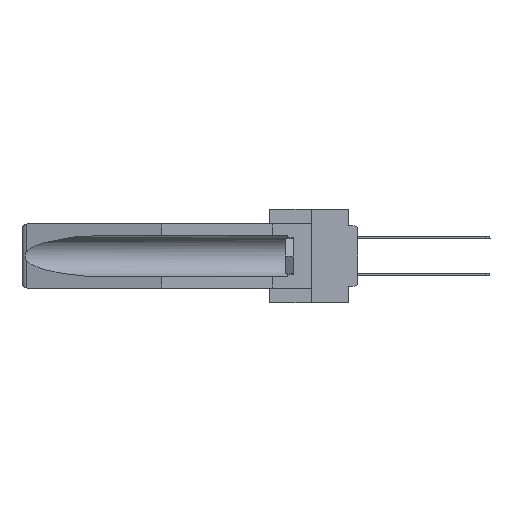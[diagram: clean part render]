
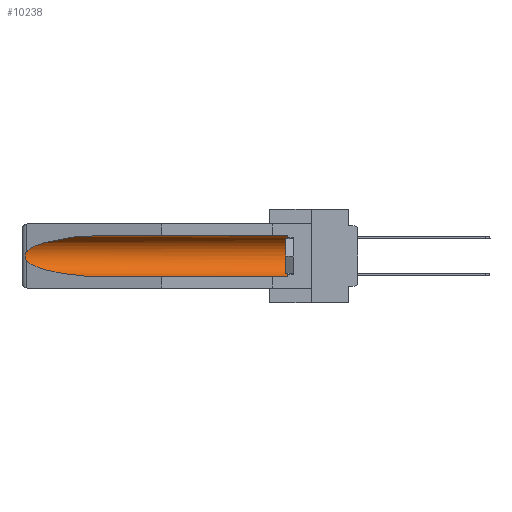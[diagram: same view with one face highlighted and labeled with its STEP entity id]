
A CAD part, left-side view. The second image highlights one B-rep face of the part: STEP entity #10238.
In plain terms, the highlighted cylindrical face has radius 2.857 mm (diameter 5.715 mm), a partial arc.
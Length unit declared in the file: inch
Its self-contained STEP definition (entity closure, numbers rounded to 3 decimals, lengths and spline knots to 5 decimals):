
#46 = EDGE_LOOP ( 'NONE', ( #25055, #23466, #17663, #6722, #11705, #9117 ) ) ;
#323 = AXIS2_PLACEMENT_3D ( 'NONE', #9166, #14554, #29353 ) ;
#663 = VECTOR ( 'NONE', #30171, 39.37008 ) ;
#1016 = CARTESIAN_POINT ( 'NONE',  ( 0.26537, 1.52718, -0.19328 ) ) ;
#2101 = DIRECTION ( 'NONE',  ( 0., 1., 0. ) ) ;
#3314 = CARTESIAN_POINT ( 'NONE',  ( 0.155, -0.30754, -0.284 ) ) ;
#3379 = VECTOR ( 'NONE', #2101, 39.37008 ) ;
#4280 =( BOUNDED_CURVE ( )  B_SPLINE_CURVE ( 3, ( #18358, #13815, #28750, #16086 ),
 .UNSPECIFIED., .F., .T. ) 
 B_SPLINE_CURVE_WITH_KNOTS ( ( 4, 4 ),
 ( 4.71239, 6.08839 ),
 .UNSPECIFIED. ) 
 CURVE ( )  GEOMETRIC_REPRESENTATION_ITEM ( )  RATIONAL_B_SPLINE_CURVE ( ( 1., 0.848, 0.848, 1. ) ) 
 REPRESENTATION_ITEM ( '' )  );
#4795 = CARTESIAN_POINT ( 'NONE',  ( 0.2675, 1.53308, -0.17534 ) ) ;
#5917 = EDGE_CURVE ( 'NONE', #19078, #24408, #18412, .T. ) ;
#6722 = ORIENTED_EDGE ( 'NONE', *, *, #12172, .F. ) ;
#9117 = ORIENTED_EDGE ( 'NONE', *, *, #14788, .T. ) ;
#9166 = CARTESIAN_POINT ( 'NONE',  ( 0.155, 0.126, -0.1715 ) ) ;
#10238 = ADVANCED_FACE ( 'NONE', ( #21677 ), #19865, .F. ) ;
#11245 = CARTESIAN_POINT ( 'NONE',  ( 0.21114, 1.30732, -0.284 ) ) ;
#11557 = CARTESIAN_POINT ( 'NONE',  ( 0.26537, 1.52718, -0.19328 ) ) ;
#11705 = ORIENTED_EDGE ( 'NONE', *, *, #15623, .T. ) ;
#12172 = EDGE_CURVE ( 'NONE', #29720, #23252, #22538, .T. ) ;
#13815 = CARTESIAN_POINT ( 'NONE',  ( 0.21114, 1.30732, -0.059 ) ) ;
#14375 = CIRCLE ( 'NONE', #323, 0.1125 ) ;
#14478 = LINE ( 'NONE', #14799, #3379 ) ;
#14554 = DIRECTION ( 'NONE',  ( 0., -1., 0. ) ) ;
#14788 = EDGE_CURVE ( 'NONE', #26849, #15546, #14478, .T. ) ;
#14799 = CARTESIAN_POINT ( 'NONE',  ( 0.155, -0.30754, -0.059 ) ) ;
#15546 = VERTEX_POINT ( 'NONE', #28231 ) ;
#15623 = EDGE_CURVE ( 'NONE', #29720, #26849, #14375, .T. ) ;
#16086 = CARTESIAN_POINT ( 'NONE',  ( 0.26537, 1.52718, -0.14972 ) ) ;
#16120 = CARTESIAN_POINT ( 'NONE',  ( 0.155, 1.07973, -0.284 ) ) ;
#16335 = EDGE_CURVE ( 'NONE', #15546, #19078, #4280, .T. ) ;
#17203 = CARTESIAN_POINT ( 'NONE',  ( 0.26654, 1.53092, -0.15636 ) ) ;
#17396 = CARTESIAN_POINT ( 'NONE',  ( 0.155, 1.07973, -0.284 ) ) ;
#17663 = ORIENTED_EDGE ( 'NONE', *, *, #23042, .T. ) ;
#17802 =( BOUNDED_CURVE ( )  B_SPLINE_CURVE ( 3, ( #11557, #26660, #11245, #16120 ),
 .UNSPECIFIED., .F., .T. ) 
 B_SPLINE_CURVE_WITH_KNOTS ( ( 4, 4 ),
 ( 0.1948, 1.5708 ),
 .UNSPECIFIED. ) 
 CURVE ( )  GEOMETRIC_REPRESENTATION_ITEM ( )  RATIONAL_B_SPLINE_CURVE ( ( 1., 0.848, 0.848, 1. ) ) 
 REPRESENTATION_ITEM ( '' )  );
#18046 = CARTESIAN_POINT ( 'NONE',  ( 0.155, 0.126, -0.059 ) ) ;
#18358 = CARTESIAN_POINT ( 'NONE',  ( 0.155, 1.07973, -0.059 ) ) ;
#18412 = B_SPLINE_CURVE_WITH_KNOTS ( 'NONE', 3,
 ( #20285, #22400, #17203, #27116, #19973, #4795, #25145, #22559, #27756, #22239 ),
 .UNSPECIFIED., .F., .F.,
 ( 4, 2, 2, 2, 4 ),
 ( 0., 0.00029, 0.00058, 0.00087, 0.00117 ),
 .UNSPECIFIED. ) ;
#19078 = VERTEX_POINT ( 'NONE', #19214 ) ;
#19214 = CARTESIAN_POINT ( 'NONE',  ( 0.26537, 1.52718, -0.14972 ) ) ;
#19865 = CYLINDRICAL_SURFACE ( 'NONE', #31056, 0.1125 ) ;
#19973 = CARTESIAN_POINT ( 'NONE',  ( 0.2675, 1.53308, -0.16763 ) ) ;
#20285 = CARTESIAN_POINT ( 'NONE',  ( 0.26537, 1.52718, -0.14972 ) ) ;
#21677 = FACE_OUTER_BOUND ( 'NONE', #46, .T. ) ;
#22239 = CARTESIAN_POINT ( 'NONE',  ( 0.26537, 1.52718, -0.19328 ) ) ;
#22400 = CARTESIAN_POINT ( 'NONE',  ( 0.26597, 1.52961, -0.15275 ) ) ;
#22538 = LINE ( 'NONE', #3314, #663 ) ;
#22559 = CARTESIAN_POINT ( 'NONE',  ( 0.26655, 1.53094, -0.18657 ) ) ;
#23042 = EDGE_CURVE ( 'NONE', #24408, #23252, #17802, .T. ) ;
#23252 = VERTEX_POINT ( 'NONE', #17396 ) ;
#23466 = ORIENTED_EDGE ( 'NONE', *, *, #5917, .T. ) ;
#24408 = VERTEX_POINT ( 'NONE', #1016 ) ;
#25055 = ORIENTED_EDGE ( 'NONE', *, *, #16335, .T. ) ;
#25145 = CARTESIAN_POINT ( 'NONE',  ( 0.2673, 1.53269, -0.17917 ) ) ;
#26660 = CARTESIAN_POINT ( 'NONE',  ( 0.25451, 1.48313, -0.24835 ) ) ;
#26684 = CARTESIAN_POINT ( 'NONE',  ( 0.155, -0.30754, -0.1715 ) ) ;
#26849 = VERTEX_POINT ( 'NONE', #18046 ) ;
#27116 = CARTESIAN_POINT ( 'NONE',  ( 0.2673, 1.5327, -0.16383 ) ) ;
#27756 = CARTESIAN_POINT ( 'NONE',  ( 0.26597, 1.5296, -0.19026 ) ) ;
#28231 = CARTESIAN_POINT ( 'NONE',  ( 0.155, 1.07973, -0.059 ) ) ;
#28750 = CARTESIAN_POINT ( 'NONE',  ( 0.25451, 1.48313, -0.09465 ) ) ;
#29353 = DIRECTION ( 'NONE',  ( 0., 0., 1. ) ) ;
#29720 = VERTEX_POINT ( 'NONE', #31673 ) ;
#30171 = DIRECTION ( 'NONE',  ( 0., 1., 0. ) ) ;
#31056 = AXIS2_PLACEMENT_3D ( 'NONE', #26684, #31559, #31875 ) ;
#31559 = DIRECTION ( 'NONE',  ( 0., 1., 0. ) ) ;
#31673 = CARTESIAN_POINT ( 'NONE',  ( 0.155, 0.126, -0.284 ) ) ;
#31875 = DIRECTION ( 'NONE',  ( 0., 0., 1. ) ) ;
